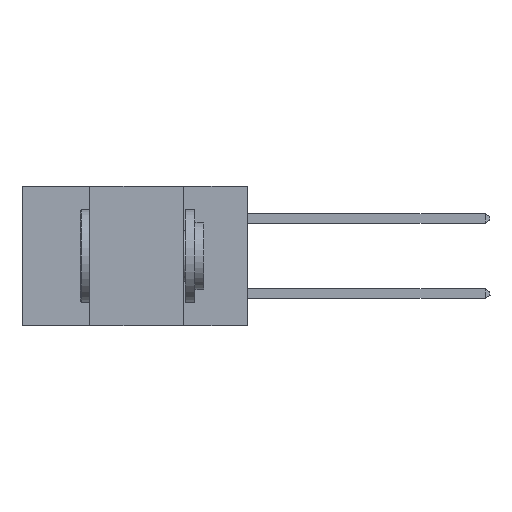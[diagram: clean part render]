
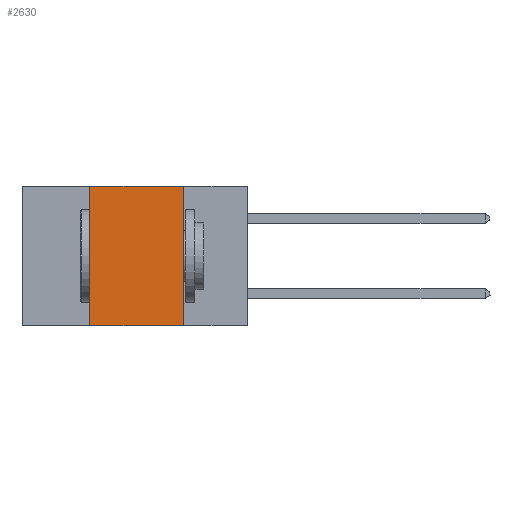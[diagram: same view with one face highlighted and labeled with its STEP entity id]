
A CAD part, left-side view. The second image highlights one B-rep face of the part: STEP entity #2630.
In plain terms, the highlighted planar face has unit normal (-1, 0, 0).
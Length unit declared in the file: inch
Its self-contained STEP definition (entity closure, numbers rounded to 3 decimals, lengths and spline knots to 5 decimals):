
#978 = VERTEX_POINT ( 'NONE', #10540 ) ;
#2262 = DIRECTION ( 'NONE',  ( 0., -1., 0. ) ) ;
#2630 = ADVANCED_FACE ( 'NONE', ( #10572 ), #10547, .F. ) ;
#3927 = LINE ( 'NONE', #13830, #20787 ) ;
#4912 = ORIENTED_EDGE ( 'NONE', *, *, #15963, .F. ) ;
#5305 = ORIENTED_EDGE ( 'NONE', *, *, #21248, .F. ) ;
#5609 = CARTESIAN_POINT ( 'NONE',  ( 0., 0.17, 0. ) ) ;
#7540 = LINE ( 'NONE', #23332, #9338 ) ;
#8439 = VERTEX_POINT ( 'NONE', #13313 ) ;
#8611 = EDGE_CURVE ( 'NONE', #16895, #8439, #7540, .T. ) ;
#9338 = VECTOR ( 'NONE', #17418, 39.37008 ) ;
#10540 = CARTESIAN_POINT ( 'NONE',  ( 0., 0.42, 0. ) ) ;
#10547 = PLANE ( 'NONE',  #22810 ) ;
#10572 = FACE_OUTER_BOUND ( 'NONE', #13140, .T. ) ;
#10870 = DIRECTION ( 'NONE',  ( 0., 0., -1. ) ) ;
#11431 = VECTOR ( 'NONE', #23798, 39.37008 ) ;
#12460 = VERTEX_POINT ( 'NONE', #5609 ) ;
#12922 = LINE ( 'NONE', #14203, #11431 ) ;
#13140 = EDGE_LOOP ( 'NONE', ( #5305, #14253, #4912, #21645 ) ) ;
#13313 = CARTESIAN_POINT ( 'NONE',  ( 0., 0.17, -0.37 ) ) ;
#13830 = CARTESIAN_POINT ( 'NONE',  ( 0., 0.6, 0. ) ) ;
#14203 = CARTESIAN_POINT ( 'NONE',  ( 0., 0.17, 0. ) ) ;
#14253 = ORIENTED_EDGE ( 'NONE', *, *, #14869, .F. ) ;
#14276 = CARTESIAN_POINT ( 'NONE',  ( 0., 0.42, -0.37 ) ) ;
#14869 = EDGE_CURVE ( 'NONE', #978, #12460, #3927, .T. ) ;
#15963 = EDGE_CURVE ( 'NONE', #16895, #978, #17078, .T. ) ;
#16327 = CARTESIAN_POINT ( 'NONE',  ( 0., 0.6, 0. ) ) ;
#16895 = VERTEX_POINT ( 'NONE', #14276 ) ;
#17078 = LINE ( 'NONE', #21517, #22554 ) ;
#17418 = DIRECTION ( 'NONE',  ( 0., -1., 0. ) ) ;
#18265 = DIRECTION ( 'NONE',  ( 1., 0., 0. ) ) ;
#20787 = VECTOR ( 'NONE', #2262, 39.37008 ) ;
#21237 = DIRECTION ( 'NONE',  ( 0., 0., 1. ) ) ;
#21248 = EDGE_CURVE ( 'NONE', #12460, #8439, #12922, .T. ) ;
#21517 = CARTESIAN_POINT ( 'NONE',  ( 0., 0.42, 0. ) ) ;
#21645 = ORIENTED_EDGE ( 'NONE', *, *, #8611, .T. ) ;
#22554 = VECTOR ( 'NONE', #21237, 39.37008 ) ;
#22810 = AXIS2_PLACEMENT_3D ( 'NONE', #16327, #18265, #10870 ) ;
#23332 = CARTESIAN_POINT ( 'NONE',  ( 0., 0.6, -0.37 ) ) ;
#23798 = DIRECTION ( 'NONE',  ( 0., 0., -1. ) ) ;
